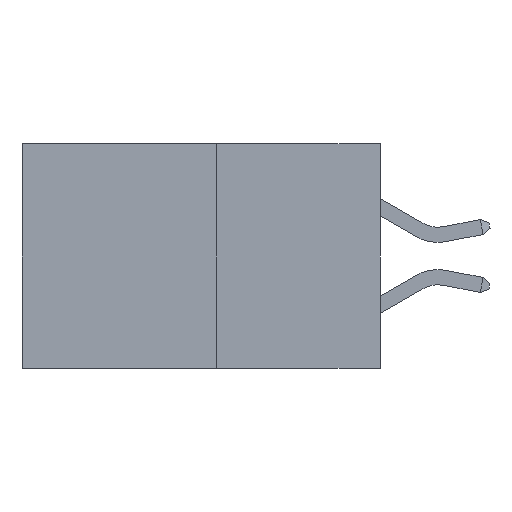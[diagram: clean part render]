
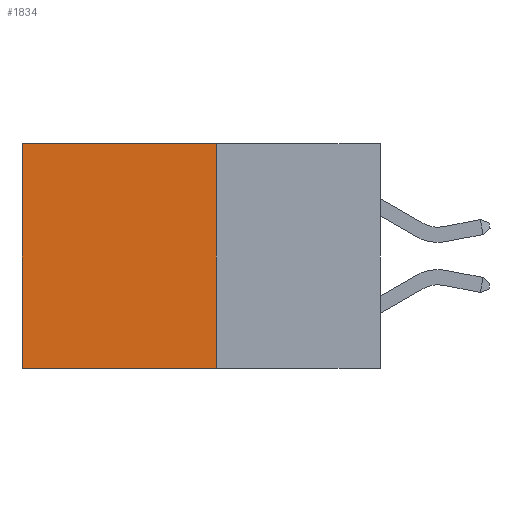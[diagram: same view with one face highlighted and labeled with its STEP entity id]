
A CAD part, left-side view. The second image highlights one B-rep face of the part: STEP entity #1834.
In plain terms, the highlighted planar face has unit normal (-1, 0, 0).
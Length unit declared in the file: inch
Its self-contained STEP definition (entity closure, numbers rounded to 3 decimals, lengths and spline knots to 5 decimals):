
#43 = DIRECTION ( 'NONE',  ( 0., 0., -1. ) ) ;
#240 = VERTEX_POINT ( 'NONE', #1454 ) ;
#1454 = CARTESIAN_POINT ( 'NONE',  ( 0.277, 0.59, -0.37 ) ) ;
#1834 = ADVANCED_FACE ( 'NONE', ( #13962 ), #24414, .F. ) ;
#2489 = DIRECTION ( 'NONE',  ( 0., 1., 0. ) ) ;
#3021 = EDGE_CURVE ( 'NONE', #21204, #5516, #6196, .T. ) ;
#3765 = DIRECTION ( 'NONE',  ( 0., 1., 0. ) ) ;
#4149 = VECTOR ( 'NONE', #43, 39.37008 ) ;
#4592 = EDGE_LOOP ( 'NONE', ( #5643, #6005, #6338, #7539 ) ) ;
#4906 = CARTESIAN_POINT ( 'NONE',  ( 0.277, 0.27, -0.37 ) ) ;
#5516 = VERTEX_POINT ( 'NONE', #4906 ) ;
#5643 = ORIENTED_EDGE ( 'NONE', *, *, #18759, .T. ) ;
#5696 = VECTOR ( 'NONE', #2489, 39.37008 ) ;
#5781 = VECTOR ( 'NONE', #3765, 39.37008 ) ;
#6005 = ORIENTED_EDGE ( 'NONE', *, *, #20917, .F. ) ;
#6196 = LINE ( 'NONE', #27812, #23286 ) ;
#6338 = ORIENTED_EDGE ( 'NONE', *, *, #3021, .F. ) ;
#6424 = LINE ( 'NONE', #11458, #5696 ) ;
#7539 = ORIENTED_EDGE ( 'NONE', *, *, #26312, .T. ) ;
#11458 = CARTESIAN_POINT ( 'NONE',  ( 0.277, 0.27, -0.37 ) ) ;
#11754 = LINE ( 'NONE', #14910, #5781 ) ;
#13645 = CARTESIAN_POINT ( 'NONE',  ( 0.277, 0.27, 0. ) ) ;
#13962 = FACE_OUTER_BOUND ( 'NONE', #4592, .T. ) ;
#14665 = AXIS2_PLACEMENT_3D ( 'NONE', #24378, #16313, #16212 ) ;
#14910 = CARTESIAN_POINT ( 'NONE',  ( 0.277, 0.27, 0. ) ) ;
#15206 = VERTEX_POINT ( 'NONE', #23757 ) ;
#16212 = DIRECTION ( 'NONE',  ( 0., 0., -1. ) ) ;
#16313 = DIRECTION ( 'NONE',  ( 1., 0., 0. ) ) ;
#18759 = EDGE_CURVE ( 'NONE', #15206, #240, #21995, .T. ) ;
#20917 = EDGE_CURVE ( 'NONE', #5516, #240, #6424, .T. ) ;
#21204 = VERTEX_POINT ( 'NONE', #13645 ) ;
#21995 = LINE ( 'NONE', #26797, #4149 ) ;
#23286 = VECTOR ( 'NONE', #28001, 39.37008 ) ;
#23757 = CARTESIAN_POINT ( 'NONE',  ( 0.277, 0.59, 0. ) ) ;
#24378 = CARTESIAN_POINT ( 'NONE',  ( 0.277, 0.27, -0.37 ) ) ;
#24414 = PLANE ( 'NONE',  #14665 ) ;
#26312 = EDGE_CURVE ( 'NONE', #21204, #15206, #11754, .T. ) ;
#26797 = CARTESIAN_POINT ( 'NONE',  ( 0.277, 0.59, -0.37 ) ) ;
#27812 = CARTESIAN_POINT ( 'NONE',  ( 0.277, 0.27, -0.37 ) ) ;
#28001 = DIRECTION ( 'NONE',  ( 0., 0., -1. ) ) ;
